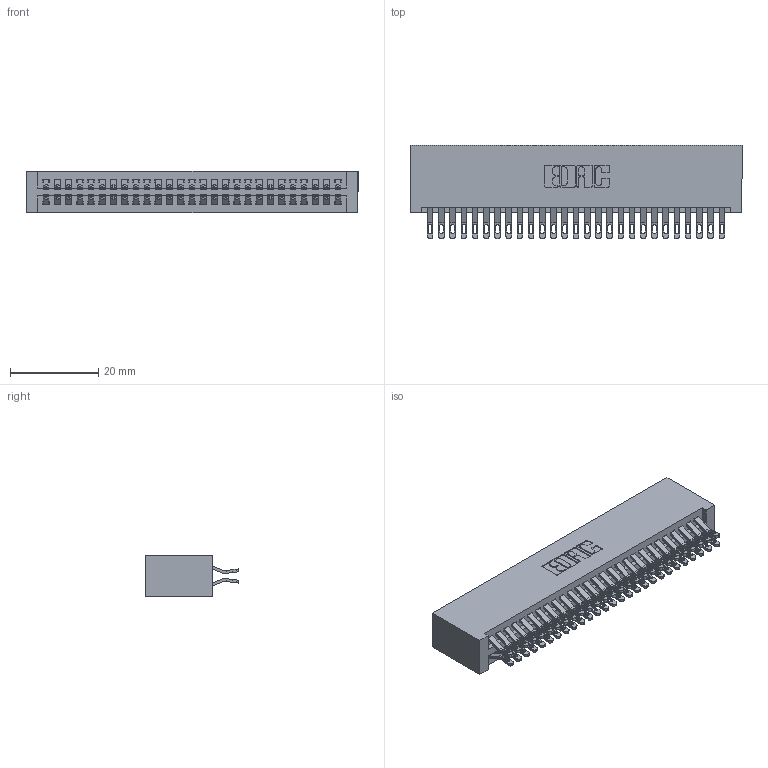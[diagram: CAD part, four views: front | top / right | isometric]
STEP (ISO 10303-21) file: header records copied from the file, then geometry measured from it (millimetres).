
FILE_DESCRIPTION (( 'STEP AP203' ), '1' );
FILE_NAME ('395-054-555-201.STEP', '2018-11-21T11:10:14', ( '' ), ( '' ), 'SwSTEP 2.0', 'SolidWorks 2016', '' );
FILE_SCHEMA (( 'CONFIG_CONTROL_DESIGN' ));
Length unit declared in the file: inch
Products named in the file (3): 345-292-001_555 Tail; 345 Part_No Mounting Lugs; 395-054-555-201
Assembly tree (55 placements, depth 2):
  395-054-555-201
    345 Part_No Mounting Lugs
    345-292-001_555 Tail  x54
Bounding box: 75.18 x 21.13 x 9.4 mm (x, y, z)
Volume: 7936.8 mm3; surface area: 12289.4 mm2
Topology: 55 solids, 55 shells, 3142 faces, 9875 edges, 6582 vertices
Faces by surface type: plane 1750, cylinder 1392
Entity records: 23253 total; most frequent: CARTESIAN_POINT 3946, ORIENTED_EDGE 3850, DIRECTION 3461, EDGE_CURVE 1925, VECTOR 1673, LINE 1673, VERTEX_POINT 1282, AXIS2_PLACEMENT_3D 894
